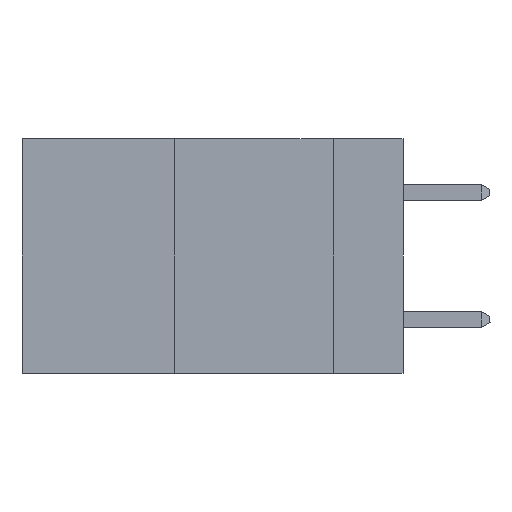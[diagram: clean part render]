
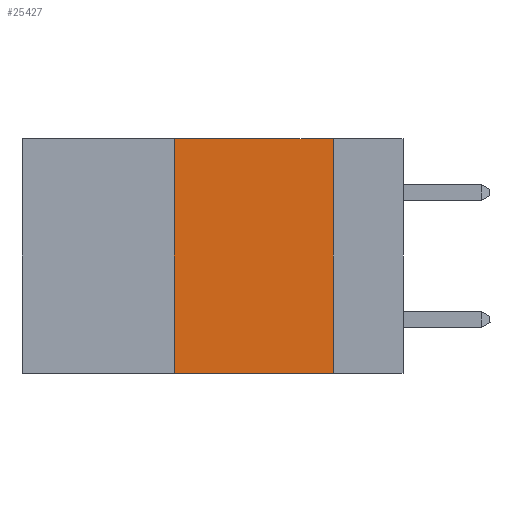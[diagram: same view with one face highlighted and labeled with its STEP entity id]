
A CAD part, left-side view. The second image highlights one B-rep face of the part: STEP entity #25427.
In plain terms, the highlighted planar face has unit normal (-1, 0, 0).
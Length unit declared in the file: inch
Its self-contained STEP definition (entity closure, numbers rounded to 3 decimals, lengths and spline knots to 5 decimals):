
#386 = LINE ( 'NONE', #6628, #47283 ) ;
#844 = ORIENTED_EDGE ( 'NONE', *, *, #32598, .F. ) ;
#3161 = ORIENTED_EDGE ( 'NONE', *, *, #30157, .F. ) ;
#6628 = CARTESIAN_POINT ( 'NONE',  ( 0., 0.6, -0.37 ) ) ;
#7997 = CARTESIAN_POINT ( 'NONE',  ( 0., 0.6, 0. ) ) ;
#9732 = FACE_OUTER_BOUND ( 'NONE', #21162, .T. ) ;
#10443 = LINE ( 'NONE', #47321, #30121 ) ;
#11857 = VECTOR ( 'NONE', #46941, 39.37008 ) ;
#14479 = VERTEX_POINT ( 'NONE', #29685 ) ;
#15384 = DIRECTION ( 'NONE',  ( 1., 0., 0. ) ) ;
#21162 = EDGE_LOOP ( 'NONE', ( #42196, #3161, #844, #23482 ) ) ;
#22800 = LINE ( 'NONE', #32019, #11857 ) ;
#23482 = ORIENTED_EDGE ( 'NONE', *, *, #26545, .T. ) ;
#23715 = VERTEX_POINT ( 'NONE', #33346 ) ;
#23963 = VERTEX_POINT ( 'NONE', #31046 ) ;
#24139 = CARTESIAN_POINT ( 'NONE',  ( 0., 0.6, 0. ) ) ;
#25001 = DIRECTION ( 'NONE',  ( 0., -1., 0. ) ) ;
#25083 = DIRECTION ( 'NONE',  ( 0., 0., -1. ) ) ;
#25427 = ADVANCED_FACE ( 'NONE', ( #9732 ), #37569, .F. ) ;
#26545 = EDGE_CURVE ( 'NONE', #23963, #30038, #386, .T. ) ;
#27866 = DIRECTION ( 'NONE',  ( 0., -1., 0. ) ) ;
#29685 = CARTESIAN_POINT ( 'NONE',  ( 0., 0.11, 0. ) ) ;
#30038 = VERTEX_POINT ( 'NONE', #30829 ) ;
#30121 = VECTOR ( 'NONE', #25083, 39.37008 ) ;
#30157 = EDGE_CURVE ( 'NONE', #23715, #14479, #31714, .T. ) ;
#30829 = CARTESIAN_POINT ( 'NONE',  ( 0., 0.11, -0.37 ) ) ;
#31046 = CARTESIAN_POINT ( 'NONE',  ( 0., 0.36, -0.37 ) ) ;
#31714 = LINE ( 'NONE', #24139, #40414 ) ;
#32019 = CARTESIAN_POINT ( 'NONE',  ( 0., 0.36, 0. ) ) ;
#32439 = AXIS2_PLACEMENT_3D ( 'NONE', #7997, #15384, #41315 ) ;
#32598 = EDGE_CURVE ( 'NONE', #23963, #23715, #22800, .T. ) ;
#33346 = CARTESIAN_POINT ( 'NONE',  ( 0., 0.36, 0. ) ) ;
#36642 = EDGE_CURVE ( 'NONE', #14479, #30038, #10443, .T. ) ;
#37569 = PLANE ( 'NONE',  #32439 ) ;
#40414 = VECTOR ( 'NONE', #27866, 39.37008 ) ;
#41315 = DIRECTION ( 'NONE',  ( 0., 0., -1. ) ) ;
#42196 = ORIENTED_EDGE ( 'NONE', *, *, #36642, .F. ) ;
#46941 = DIRECTION ( 'NONE',  ( 0., 0., 1. ) ) ;
#47283 = VECTOR ( 'NONE', #25001, 39.37008 ) ;
#47321 = CARTESIAN_POINT ( 'NONE',  ( 0., 0.11, 0. ) ) ;
